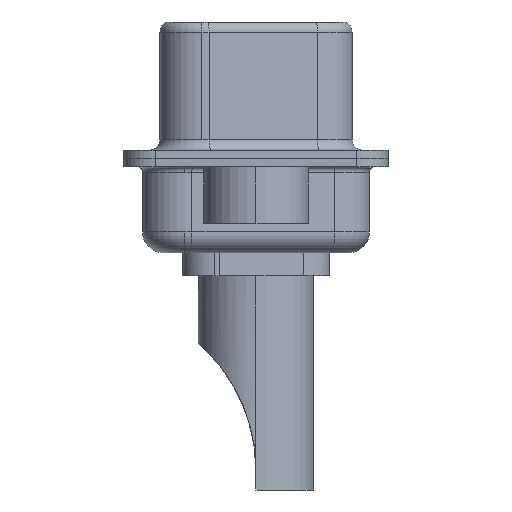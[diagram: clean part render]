
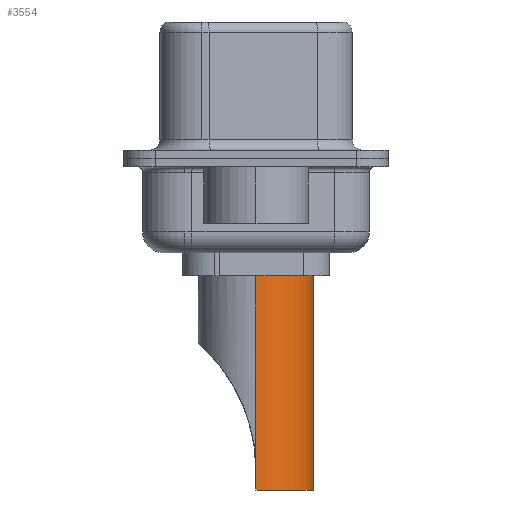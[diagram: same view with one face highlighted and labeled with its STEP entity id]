
A CAD part, left-side view. The second image highlights one B-rep face of the part: STEP entity #3554.
In plain terms, the highlighted cylindrical face has radius 2.75 mm (diameter 5.5 mm), a partial arc.
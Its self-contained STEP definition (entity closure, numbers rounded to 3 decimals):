
#13 = EDGE_CURVE ( 'NONE', #4395, #2633, #5795, .T. ) ;
#80 = EDGE_CURVE ( 'NONE', #12222, #2633, #12595, .T. ) ;
#226 = EDGE_CURVE ( 'NONE', #6841, #11087, #11700, .T. ) ;
#242 = CARTESIAN_POINT ( 'NONE',  ( 2.75, 0., 1.5 ) ) ;
#557 = LINE ( 'NONE', #5277, #4035 ) ;
#638 = DIRECTION ( 'NONE',  ( 1., 0., 0. ) ) ;
#939 = CYLINDRICAL_SURFACE ( 'NONE', #2761, 2.75 ) ;
#1168 = LINE ( 'NONE', #14282, #12270 ) ;
#1449 = ORIENTED_EDGE ( 'NONE', *, *, #80, .F. ) ;
#2327 = CARTESIAN_POINT ( 'NONE',  ( 0., 0., 1.5 ) ) ;
#2633 = VERTEX_POINT ( 'NONE', #9999 ) ;
#2761 = AXIS2_PLACEMENT_3D ( 'NONE', #3417, #8403, #638 ) ;
#3382 = LINE ( 'NONE', #4621, #10488 ) ;
#3417 = CARTESIAN_POINT ( 'NONE',  ( 0., 0., 4.234 ) ) ;
#3554 = ADVANCED_FACE ( 'NONE', ( #9025 ), #939, .T. ) ;
#3745 = ORIENTED_EDGE ( 'NONE', *, *, #226, .F. ) ;
#4035 = VECTOR ( 'NONE', #8133, 1000. ) ;
#4264 = DIRECTION ( 'NONE',  ( 0., 0., 1. ) ) ;
#4395 = VERTEX_POINT ( 'NONE', #5675 ) ;
#4621 = CARTESIAN_POINT ( 'NONE',  ( -2.75, 0., -8.7 ) ) ;
#4967 = VECTOR ( 'NONE', #13106, 1000. ) ;
#5277 = CARTESIAN_POINT ( 'NONE',  ( 2.75, 0., 4.234 ) ) ;
#5415 = ORIENTED_EDGE ( 'NONE', *, *, #17641, .T. ) ;
#5675 = CARTESIAN_POINT ( 'NONE',  ( -2.75, 0., -8.7 ) ) ;
#5795 = CIRCLE ( 'NONE', #16031, 2.75 ) ;
#6365 = EDGE_CURVE ( 'NONE', #15774, #6841, #1168, .T. ) ;
#6439 = CARTESIAN_POINT ( 'NONE',  ( 2.75, 0., -8.7 ) ) ;
#6801 = CARTESIAN_POINT ( 'NONE',  ( -2.75, 0., 1.5 ) ) ;
#6840 = DIRECTION ( 'NONE',  ( 1., 0., 0. ) ) ;
#6841 = VERTEX_POINT ( 'NONE', #6801 ) ;
#8133 = DIRECTION ( 'NONE',  ( 0., 0., 1. ) ) ;
#8403 = DIRECTION ( 'NONE',  ( 0., 0., 1. ) ) ;
#9025 = FACE_OUTER_BOUND ( 'NONE', #10381, .T. ) ;
#9028 = CARTESIAN_POINT ( 'NONE',  ( -2.75, 0., -7.764 ) ) ;
#9857 = AXIS2_PLACEMENT_3D ( 'NONE', #2327, #14666, #14726 ) ;
#9999 = CARTESIAN_POINT ( 'NONE',  ( 2.75, 0., -8.7 ) ) ;
#10381 = EDGE_LOOP ( 'NONE', ( #16414, #5415, #13532, #1449, #16726, #3745 ) ) ;
#10488 = VECTOR ( 'NONE', #11830, 1000. ) ;
#10637 = CARTESIAN_POINT ( 'NONE',  ( 2.75, 0., -7.764 ) ) ;
#11087 = VERTEX_POINT ( 'NONE', #242 ) ;
#11700 = CIRCLE ( 'NONE', #9857, 2.75 ) ;
#11830 = DIRECTION ( 'NONE',  ( 0., 0., -1. ) ) ;
#12222 = VERTEX_POINT ( 'NONE', #10637 ) ;
#12270 = VECTOR ( 'NONE', #4264, 1000. ) ;
#12423 = CARTESIAN_POINT ( 'NONE',  ( 0., 0., -8.7 ) ) ;
#12595 = LINE ( 'NONE', #6439, #4967 ) ;
#13106 = DIRECTION ( 'NONE',  ( 0., 0., -1. ) ) ;
#13532 = ORIENTED_EDGE ( 'NONE', *, *, #13, .T. ) ;
#14123 = DIRECTION ( 'NONE',  ( 0., 0., 1. ) ) ;
#14282 = CARTESIAN_POINT ( 'NONE',  ( -2.75, 0., 4.234 ) ) ;
#14666 = DIRECTION ( 'NONE',  ( 0., 0., 1. ) ) ;
#14726 = DIRECTION ( 'NONE',  ( 1., 0., 0. ) ) ;
#15774 = VERTEX_POINT ( 'NONE', #9028 ) ;
#16031 = AXIS2_PLACEMENT_3D ( 'NONE', #12423, #14123, #6840 ) ;
#16414 = ORIENTED_EDGE ( 'NONE', *, *, #6365, .F. ) ;
#16726 = ORIENTED_EDGE ( 'NONE', *, *, #17322, .T. ) ;
#17322 = EDGE_CURVE ( 'NONE', #12222, #11087, #557, .T. ) ;
#17641 = EDGE_CURVE ( 'NONE', #15774, #4395, #3382, .T. ) ;
